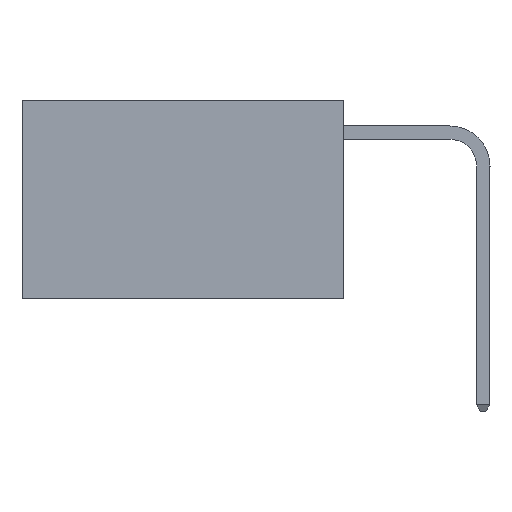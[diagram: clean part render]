
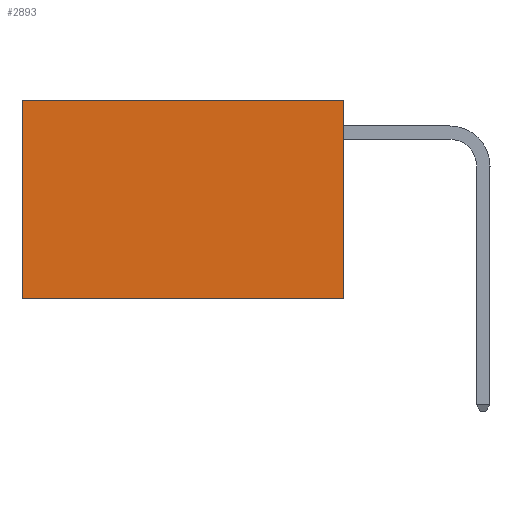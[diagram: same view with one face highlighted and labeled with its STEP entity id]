
A CAD part, left-side view. The second image highlights one B-rep face of the part: STEP entity #2893.
In plain terms, the highlighted planar face has unit normal (-1, 0, 0).
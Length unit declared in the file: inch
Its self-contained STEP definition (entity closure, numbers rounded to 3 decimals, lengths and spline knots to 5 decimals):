
#394 = ORIENTED_EDGE ( 'NONE', *, *, #11080, .F. ) ;
#961 = PLANE ( 'NONE',  #16502 ) ;
#963 = DIRECTION ( 'NONE',  ( 0., 1., 0. ) ) ;
#1116 = CARTESIAN_POINT ( 'NONE',  ( 0.2625, 0., 0. ) ) ;
#1182 = EDGE_LOOP ( 'NONE', ( #12568, #394, #3551, #8023 ) ) ;
#1320 = DIRECTION ( 'NONE',  ( 1., 0., 0. ) ) ;
#1986 = DIRECTION ( 'NONE',  ( 0., 0., -1. ) ) ;
#2013 = CARTESIAN_POINT ( 'NONE',  ( 0.2625, 0., 0. ) ) ;
#2629 = CARTESIAN_POINT ( 'NONE',  ( 0.2625, 0.6, 0. ) ) ;
#2810 = VERTEX_POINT ( 'NONE', #2629 ) ;
#2893 = ADVANCED_FACE ( 'NONE', ( #5177 ), #961, .F. ) ;
#3344 = EDGE_CURVE ( 'NONE', #5929, #10259, #8468, .T. ) ;
#3394 = CARTESIAN_POINT ( 'NONE',  ( 0.2625, 0.6, 0. ) ) ;
#3551 = ORIENTED_EDGE ( 'NONE', *, *, #3344, .F. ) ;
#4255 = DIRECTION ( 'NONE',  ( 0., 0., -1. ) ) ;
#4312 = VECTOR ( 'NONE', #14587, 39.37008 ) ;
#4486 = LINE ( 'NONE', #6219, #8232 ) ;
#4726 = VECTOR ( 'NONE', #1986, 39.37008 ) ;
#5177 = FACE_OUTER_BOUND ( 'NONE', #1182, .T. ) ;
#5929 = VERTEX_POINT ( 'NONE', #2013 ) ;
#6219 = CARTESIAN_POINT ( 'NONE',  ( 0.2625, 0., -0.37 ) ) ;
#6359 = CARTESIAN_POINT ( 'NONE',  ( 0.2625, 0., 0. ) ) ;
#6761 = EDGE_CURVE ( 'NONE', #5929, #2810, #6804, .T. ) ;
#6804 = LINE ( 'NONE', #17648, #9647 ) ;
#8023 = ORIENTED_EDGE ( 'NONE', *, *, #6761, .T. ) ;
#8232 = VECTOR ( 'NONE', #10441, 39.37008 ) ;
#8468 = LINE ( 'NONE', #6359, #4726 ) ;
#9373 = VERTEX_POINT ( 'NONE', #10386 ) ;
#9647 = VECTOR ( 'NONE', #963, 39.37008 ) ;
#10002 = EDGE_CURVE ( 'NONE', #2810, #9373, #10237, .T. ) ;
#10237 = LINE ( 'NONE', #3394, #4312 ) ;
#10259 = VERTEX_POINT ( 'NONE', #12770 ) ;
#10386 = CARTESIAN_POINT ( 'NONE',  ( 0.2625, 0.6, -0.37 ) ) ;
#10441 = DIRECTION ( 'NONE',  ( 0., 1., 0. ) ) ;
#11080 = EDGE_CURVE ( 'NONE', #10259, #9373, #4486, .T. ) ;
#12568 = ORIENTED_EDGE ( 'NONE', *, *, #10002, .T. ) ;
#12770 = CARTESIAN_POINT ( 'NONE',  ( 0.2625, 0., -0.37 ) ) ;
#14587 = DIRECTION ( 'NONE',  ( 0., 0., -1. ) ) ;
#16502 = AXIS2_PLACEMENT_3D ( 'NONE', #1116, #1320, #4255 ) ;
#17648 = CARTESIAN_POINT ( 'NONE',  ( 0.2625, 0., 0. ) ) ;
